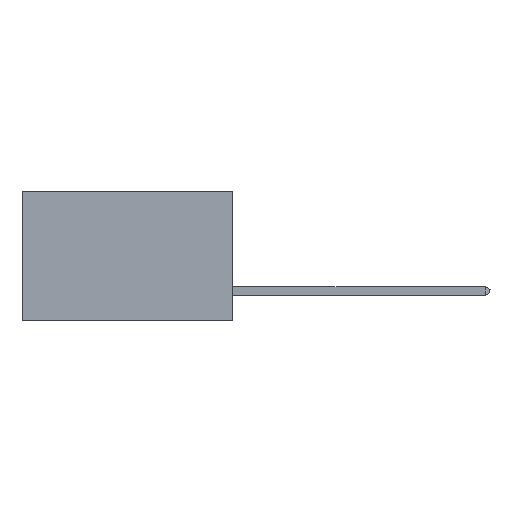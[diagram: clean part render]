
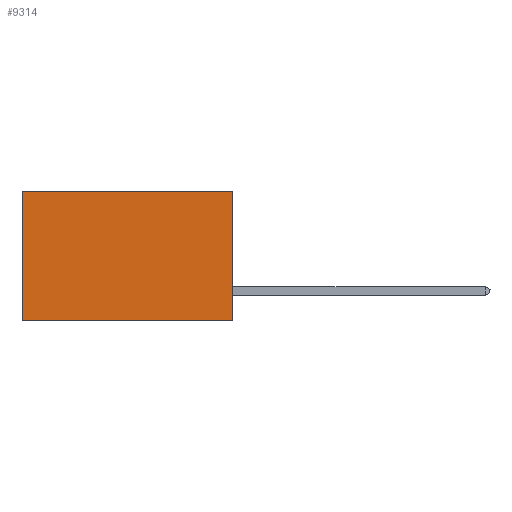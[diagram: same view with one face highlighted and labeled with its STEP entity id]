
A CAD part, left-side view. The second image highlights one B-rep face of the part: STEP entity #9314.
In plain terms, the highlighted planar face has unit normal (-1, 0, 0).
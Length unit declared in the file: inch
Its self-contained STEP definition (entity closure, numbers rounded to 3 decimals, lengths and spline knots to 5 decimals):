
#578 = VECTOR ( 'NONE', #20626, 39.37008 ) ;
#782 = FACE_OUTER_BOUND ( 'NONE', #14032, .T. ) ;
#1091 = CARTESIAN_POINT ( 'NONE',  ( 0.2875, 0.6, -0.37 ) ) ;
#3057 = PLANE ( 'NONE',  #23216 ) ;
#5149 = DIRECTION ( 'NONE',  ( 0., 0., -1. ) ) ;
#5865 = CARTESIAN_POINT ( 'NONE',  ( 0.2875, 0., 0. ) ) ;
#8603 = DIRECTION ( 'NONE',  ( 0., 0., -1. ) ) ;
#9314 = ADVANCED_FACE ( 'NONE', ( #782 ), #3057, .F. ) ;
#10249 = CARTESIAN_POINT ( 'NONE',  ( 0.2875, 0., 0. ) ) ;
#10331 = LINE ( 'NONE', #12050, #578 ) ;
#10531 = VERTEX_POINT ( 'NONE', #15109 ) ;
#10617 = DIRECTION ( 'NONE',  ( 0., 0., -1. ) ) ;
#11143 = CARTESIAN_POINT ( 'NONE',  ( 0.2875, 0., 0. ) ) ;
#11300 = VECTOR ( 'NONE', #20649, 39.37008 ) ;
#12050 = CARTESIAN_POINT ( 'NONE',  ( 0.2875, 0., -0.37 ) ) ;
#12611 = EDGE_CURVE ( 'NONE', #10531, #16598, #13778, .T. ) ;
#13155 = EDGE_CURVE ( 'NONE', #16886, #16598, #10331, .T. ) ;
#13778 = LINE ( 'NONE', #17425, #22664 ) ;
#13969 = ORIENTED_EDGE ( 'NONE', *, *, #13155, .F. ) ;
#14032 = EDGE_LOOP ( 'NONE', ( #18305, #13969, #18675, #18795 ) ) ;
#15109 = CARTESIAN_POINT ( 'NONE',  ( 0.2875, 0.6, 0. ) ) ;
#16598 = VERTEX_POINT ( 'NONE', #1091 ) ;
#16753 = LINE ( 'NONE', #5865, #11300 ) ;
#16886 = VERTEX_POINT ( 'NONE', #20746 ) ;
#17425 = CARTESIAN_POINT ( 'NONE',  ( 0.2875, 0.6, 0. ) ) ;
#18305 = ORIENTED_EDGE ( 'NONE', *, *, #12611, .T. ) ;
#18612 = LINE ( 'NONE', #11143, #19463 ) ;
#18675 = ORIENTED_EDGE ( 'NONE', *, *, #20606, .F. ) ;
#18795 = ORIENTED_EDGE ( 'NONE', *, *, #21976, .T. ) ;
#19463 = VECTOR ( 'NONE', #10617, 39.37008 ) ;
#19503 = DIRECTION ( 'NONE',  ( 1., 0., 0. ) ) ;
#20450 = CARTESIAN_POINT ( 'NONE',  ( 0.2875, 0., 0. ) ) ;
#20606 = EDGE_CURVE ( 'NONE', #23635, #16886, #18612, .T. ) ;
#20626 = DIRECTION ( 'NONE',  ( 0., 1., 0. ) ) ;
#20649 = DIRECTION ( 'NONE',  ( 0., 1., 0. ) ) ;
#20746 = CARTESIAN_POINT ( 'NONE',  ( 0.2875, 0., -0.37 ) ) ;
#21976 = EDGE_CURVE ( 'NONE', #23635, #10531, #16753, .T. ) ;
#22664 = VECTOR ( 'NONE', #8603, 39.37008 ) ;
#23216 = AXIS2_PLACEMENT_3D ( 'NONE', #10249, #19503, #5149 ) ;
#23635 = VERTEX_POINT ( 'NONE', #20450 ) ;
